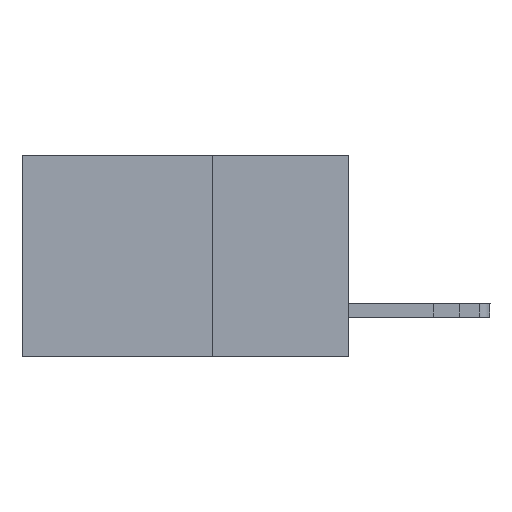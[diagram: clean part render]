
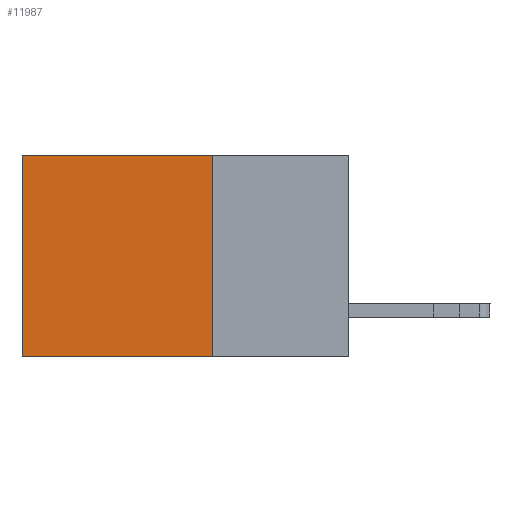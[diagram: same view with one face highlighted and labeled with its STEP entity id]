
A CAD part, left-side view. The second image highlights one B-rep face of the part: STEP entity #11987.
In plain terms, the highlighted planar face has unit normal (-1, 0, 0).
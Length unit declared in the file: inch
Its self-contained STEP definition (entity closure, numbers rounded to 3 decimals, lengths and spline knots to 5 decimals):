
#1109 = CARTESIAN_POINT ( 'NONE',  ( 0.2615, 0.25, -0.37 ) ) ;
#1466 = EDGE_CURVE ( 'NONE', #5188, #6122, #10206, .T. ) ;
#3048 = ORIENTED_EDGE ( 'NONE', *, *, #1466, .T. ) ;
#3612 = DIRECTION ( 'NONE',  ( 0., 0., -1. ) ) ;
#3704 = DIRECTION ( 'NONE',  ( 1., 0., 0. ) ) ;
#3791 = CARTESIAN_POINT ( 'NONE',  ( 0.2615, 0.25, 0. ) ) ;
#3818 = CARTESIAN_POINT ( 'NONE',  ( 0.2615, 0.6, -0.37 ) ) ;
#4020 = EDGE_CURVE ( 'NONE', #14018, #7597, #11441, .T. ) ;
#4081 = DIRECTION ( 'NONE',  ( 0., 1., 0. ) ) ;
#4704 = ORIENTED_EDGE ( 'NONE', *, *, #4020, .F. ) ;
#5188 = VERTEX_POINT ( 'NONE', #11270 ) ;
#5884 = CARTESIAN_POINT ( 'NONE',  ( 0.2615, 0.6, -0.37 ) ) ;
#6122 = VERTEX_POINT ( 'NONE', #3818 ) ;
#6778 = EDGE_CURVE ( 'NONE', #7597, #6122, #11342, .T. ) ;
#7063 = DIRECTION ( 'NONE',  ( 0., 0., -1. ) ) ;
#7158 = PLANE ( 'NONE',  #8050 ) ;
#7597 = VERTEX_POINT ( 'NONE', #14819 ) ;
#7688 = ORIENTED_EDGE ( 'NONE', *, *, #14497, .T. ) ;
#7846 = VECTOR ( 'NONE', #10744, 39.37008 ) ;
#8050 = AXIS2_PLACEMENT_3D ( 'NONE', #10714, #3704, #13070 ) ;
#9098 = VECTOR ( 'NONE', #7063, 39.37008 ) ;
#10206 = LINE ( 'NONE', #5884, #9098 ) ;
#10640 = CARTESIAN_POINT ( 'NONE',  ( 0.2615, 0.25, -0.37 ) ) ;
#10714 = CARTESIAN_POINT ( 'NONE',  ( 0.2615, 0.25, -0.37 ) ) ;
#10744 = DIRECTION ( 'NONE',  ( 0., 1., 0. ) ) ;
#10866 = VECTOR ( 'NONE', #4081, 39.37008 ) ;
#11232 = LINE ( 'NONE', #3791, #10866 ) ;
#11265 = VECTOR ( 'NONE', #3612, 39.37008 ) ;
#11270 = CARTESIAN_POINT ( 'NONE',  ( 0.2615, 0.6, 0. ) ) ;
#11342 = LINE ( 'NONE', #10640, #7846 ) ;
#11441 = LINE ( 'NONE', #1109, #11265 ) ;
#11987 = ADVANCED_FACE ( 'NONE', ( #15227 ), #7158, .F. ) ;
#11995 = CARTESIAN_POINT ( 'NONE',  ( 0.2615, 0.25, 0. ) ) ;
#12068 = EDGE_LOOP ( 'NONE', ( #3048, #12708, #4704, #7688 ) ) ;
#12708 = ORIENTED_EDGE ( 'NONE', *, *, #6778, .F. ) ;
#13070 = DIRECTION ( 'NONE',  ( 0., 0., -1. ) ) ;
#14018 = VERTEX_POINT ( 'NONE', #11995 ) ;
#14497 = EDGE_CURVE ( 'NONE', #14018, #5188, #11232, .T. ) ;
#14819 = CARTESIAN_POINT ( 'NONE',  ( 0.2615, 0.25, -0.37 ) ) ;
#15227 = FACE_OUTER_BOUND ( 'NONE', #12068, .T. ) ;
